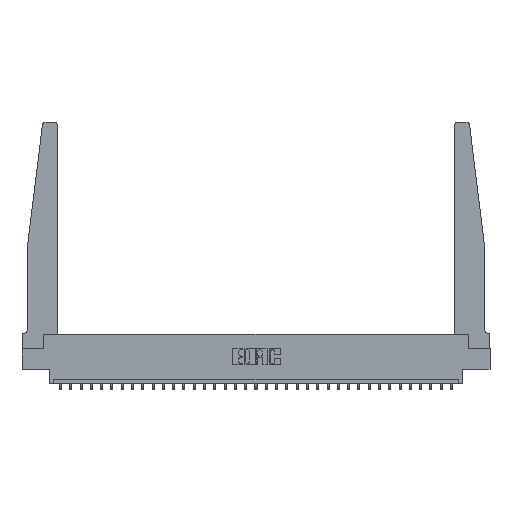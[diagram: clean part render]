
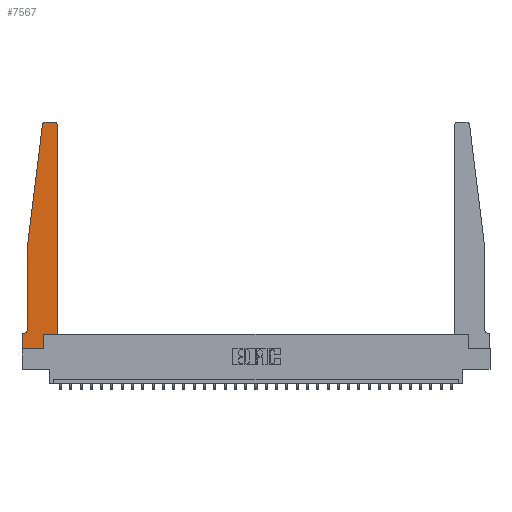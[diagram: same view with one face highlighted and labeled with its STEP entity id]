
A CAD part, top view. The second image highlights one B-rep face of the part: STEP entity #7567.
In plain terms, the highlighted planar face has unit normal (0, 0, 1).
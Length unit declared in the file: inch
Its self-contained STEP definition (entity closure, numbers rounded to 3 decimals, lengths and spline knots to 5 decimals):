
#188 = AXIS2_PLACEMENT_3D ( 'NONE', #29081, #17706, #13002 ) ;
#422 = DIRECTION ( 'NONE',  ( 1., 0., 0. ) ) ;
#558 = VERTEX_POINT ( 'NONE', #14260 ) ;
#668 = EDGE_CURVE ( 'NONE', #15828, #27071, #2179, .T. ) ;
#1082 = VERTEX_POINT ( 'NONE', #26682 ) ;
#1085 = DIRECTION ( 'NONE',  ( 0., -1., 0. ) ) ;
#1112 = ORIENTED_EDGE ( 'NONE', *, *, #29191, .T. ) ;
#1401 = VERTEX_POINT ( 'NONE', #4684 ) ;
#1498 = CARTESIAN_POINT ( 'NONE',  ( 0.065, 1.25, 0.37 ) ) ;
#1895 = EDGE_CURVE ( 'NONE', #1082, #558, #16866, .T. ) ;
#2179 = LINE ( 'NONE', #11027, #2379 ) ;
#2303 = EDGE_CURVE ( 'NONE', #558, #4328, #17272, .T. ) ;
#2379 = VECTOR ( 'NONE', #16042, 39.37008 ) ;
#2681 = EDGE_CURVE ( 'NONE', #27284, #17984, #15070, .T. ) ;
#2722 = DIRECTION ( 'NONE',  ( -1., 0., 0. ) ) ;
#2771 = AXIS2_PLACEMENT_3D ( 'NONE', #21999, #19007, #17143 ) ;
#2971 = ORIENTED_EDGE ( 'NONE', *, *, #2303, .T. ) ;
#3101 = CARTESIAN_POINT ( 'NONE',  ( 0., 0., 0.37 ) ) ;
#3437 = LINE ( 'NONE', #24443, #18509 ) ;
#3724 = CARTESIAN_POINT ( 'NONE',  ( 0., 0., 0.37 ) ) ;
#3927 = CARTESIAN_POINT ( 'NONE',  ( 0.2605, 0.18, 0.37 ) ) ;
#4328 = VERTEX_POINT ( 'NONE', #3724 ) ;
#4431 = CARTESIAN_POINT ( 'NONE',  ( 0.425, 0.18, 0.37 ) ) ;
#4684 = CARTESIAN_POINT ( 'NONE',  ( 0.2605, 0., 0.37 ) ) ;
#5529 = CARTESIAN_POINT ( 'NONE',  ( 0.25, 2.75, 0.37 ) ) ;
#5714 = EDGE_CURVE ( 'NONE', #17769, #8159, #12525, .T. ) ;
#5869 = EDGE_LOOP ( 'NONE', ( #18497, #26805, #21252, #19998, #7185, #9416, #2971, #1112, #24311, #11203, #10225, #12920 ) ) ;
#7185 = ORIENTED_EDGE ( 'NONE', *, *, #23152, .T. ) ;
#7380 = DIRECTION ( 'NONE',  ( 1., 0., 0. ) ) ;
#7567 = ADVANCED_FACE ( 'NONE', ( #26451 ), #24007, .T. ) ;
#8159 = VERTEX_POINT ( 'NONE', #10917 ) ;
#9396 = CARTESIAN_POINT ( 'NONE',  ( 0.065, 0.2375, 0.37 ) ) ;
#9416 = ORIENTED_EDGE ( 'NONE', *, *, #1895, .T. ) ;
#10225 = ORIENTED_EDGE ( 'NONE', *, *, #668, .T. ) ;
#10295 = CARTESIAN_POINT ( 'NONE',  ( 0.395, 2.72, 0.37 ) ) ;
#10471 = EDGE_CURVE ( 'NONE', #8159, #23163, #20258, .T. ) ;
#10817 = CIRCLE ( 'NONE', #19526, 0.03 ) ;
#10917 = CARTESIAN_POINT ( 'NONE',  ( 0.27653, 2.75, 0.37 ) ) ;
#11027 = CARTESIAN_POINT ( 'NONE',  ( 0.425, 0.18, 0.37 ) ) ;
#11203 = ORIENTED_EDGE ( 'NONE', *, *, #17970, .T. ) ;
#11277 = CARTESIAN_POINT ( 'NONE',  ( 0.425, 2.72, 0.37 ) ) ;
#12519 = CARTESIAN_POINT ( 'NONE',  ( 0.2605, 0.18, 0.37 ) ) ;
#12525 = LINE ( 'NONE', #5529, #25988 ) ;
#12598 = VECTOR ( 'NONE', #2722, 39.37008 ) ;
#12920 = ORIENTED_EDGE ( 'NONE', *, *, #21333, .T. ) ;
#13002 = DIRECTION ( 'NONE',  ( -1., 0., 0. ) ) ;
#13919 = EDGE_CURVE ( 'NONE', #1401, #29141, #14361, .T. ) ;
#14260 = CARTESIAN_POINT ( 'NONE',  ( 0., 0.1875, 0.37 ) ) ;
#14290 = CARTESIAN_POINT ( 'NONE',  ( 0.065, 0.1875, 0.37 ) ) ;
#14361 = LINE ( 'NONE', #12519, #20825 ) ;
#14959 = DIRECTION ( 'NONE',  ( -1., 0., 0. ) ) ;
#15070 = LINE ( 'NONE', #29171, #29185 ) ;
#15614 = CARTESIAN_POINT ( 'NONE',  ( 0., 0., 0.37 ) ) ;
#15828 = VERTEX_POINT ( 'NONE', #4431 ) ;
#16042 = DIRECTION ( 'NONE',  ( 0., 1., 0. ) ) ;
#16244 = CARTESIAN_POINT ( 'NONE',  ( 0.425, 0.18, 0.37 ) ) ;
#16866 = LINE ( 'NONE', #14290, #12598 ) ;
#17143 = DIRECTION ( 'NONE',  ( 1., 0., 0. ) ) ;
#17272 = LINE ( 'NONE', #15614, #19008 ) ;
#17451 = DIRECTION ( 'NONE',  ( 0., 0., 1. ) ) ;
#17673 = CIRCLE ( 'NONE', #188, 0.05 ) ;
#17706 = DIRECTION ( 'NONE',  ( 0., 0., -1. ) ) ;
#17769 = VERTEX_POINT ( 'NONE', #28543 ) ;
#17775 = EDGE_CURVE ( 'NONE', #23163, #27284, #3437, .T. ) ;
#17970 = EDGE_CURVE ( 'NONE', #29141, #15828, #18357, .T. ) ;
#17984 = VERTEX_POINT ( 'NONE', #9396 ) ;
#18027 = AXIS2_PLACEMENT_3D ( 'NONE', #29001, #17451, #21590 ) ;
#18357 = LINE ( 'NONE', #16244, #25827 ) ;
#18497 = ORIENTED_EDGE ( 'NONE', *, *, #5714, .T. ) ;
#18509 = VECTOR ( 'NONE', #26431, 39.37008 ) ;
#19007 = DIRECTION ( 'NONE',  ( 0., 0., 1. ) ) ;
#19008 = VECTOR ( 'NONE', #19545, 39.37008 ) ;
#19359 = LINE ( 'NONE', #3101, #20478 ) ;
#19526 = AXIS2_PLACEMENT_3D ( 'NONE', #10295, #28680, #422 ) ;
#19545 = DIRECTION ( 'NONE',  ( 0., -1., 0. ) ) ;
#19998 = ORIENTED_EDGE ( 'NONE', *, *, #2681, .T. ) ;
#20258 = CIRCLE ( 'NONE', #2771, 0.03 ) ;
#20478 = VECTOR ( 'NONE', #7380, 39.37008 ) ;
#20825 = VECTOR ( 'NONE', #23628, 39.37008 ) ;
#21252 = ORIENTED_EDGE ( 'NONE', *, *, #17775, .T. ) ;
#21333 = EDGE_CURVE ( 'NONE', #27071, #17769, #10817, .T. ) ;
#21590 = DIRECTION ( 'NONE',  ( 1., 0., 0. ) ) ;
#21999 = CARTESIAN_POINT ( 'NONE',  ( 0.27653, 2.72, 0.37 ) ) ;
#23152 = EDGE_CURVE ( 'NONE', #17984, #1082, #17673, .T. ) ;
#23163 = VERTEX_POINT ( 'NONE', #26678 ) ;
#23628 = DIRECTION ( 'NONE',  ( 0., 1., 0. ) ) ;
#24007 = PLANE ( 'NONE',  #18027 ) ;
#24311 = ORIENTED_EDGE ( 'NONE', *, *, #13919, .T. ) ;
#24443 = CARTESIAN_POINT ( 'NONE',  ( 0.065, 1.25, 0.37 ) ) ;
#25827 = VECTOR ( 'NONE', #28205, 39.37008 ) ;
#25988 = VECTOR ( 'NONE', #14959, 39.37008 ) ;
#26431 = DIRECTION ( 'NONE',  ( -0.122, -0.992, 0. ) ) ;
#26451 = FACE_OUTER_BOUND ( 'NONE', #5869, .T. ) ;
#26678 = CARTESIAN_POINT ( 'NONE',  ( 0.24675, 2.72367, 0.37 ) ) ;
#26682 = CARTESIAN_POINT ( 'NONE',  ( 0.015, 0.1875, 0.37 ) ) ;
#26805 = ORIENTED_EDGE ( 'NONE', *, *, #10471, .T. ) ;
#27071 = VERTEX_POINT ( 'NONE', #11277 ) ;
#27284 = VERTEX_POINT ( 'NONE', #1498 ) ;
#28205 = DIRECTION ( 'NONE',  ( 1., 0., 0. ) ) ;
#28543 = CARTESIAN_POINT ( 'NONE',  ( 0.395, 2.75, 0.37 ) ) ;
#28680 = DIRECTION ( 'NONE',  ( 0., 0., 1. ) ) ;
#29001 = CARTESIAN_POINT ( 'NONE',  ( 0., 0.1875, 0.37 ) ) ;
#29081 = CARTESIAN_POINT ( 'NONE',  ( 0.015, 0.2375, 0.37 ) ) ;
#29141 = VERTEX_POINT ( 'NONE', #3927 ) ;
#29171 = CARTESIAN_POINT ( 'NONE',  ( 0.065, 1.25, 0.37 ) ) ;
#29185 = VECTOR ( 'NONE', #1085, 39.37008 ) ;
#29191 = EDGE_CURVE ( 'NONE', #4328, #1401, #19359, .T. ) ;
